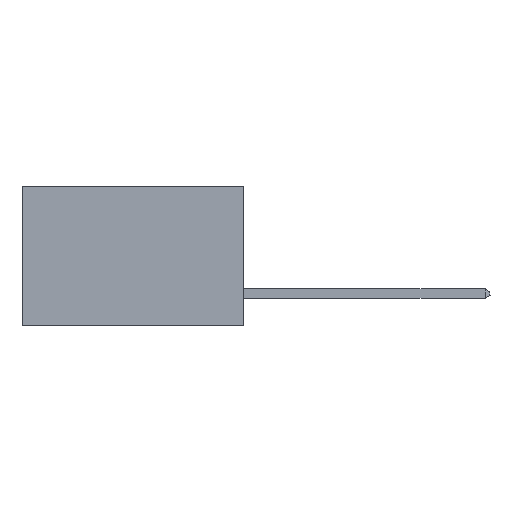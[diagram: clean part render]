
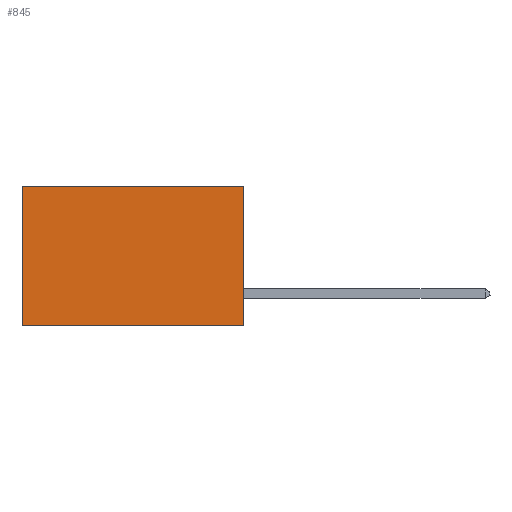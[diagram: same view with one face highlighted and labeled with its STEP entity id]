
A CAD part, left-side view. The second image highlights one B-rep face of the part: STEP entity #845.
In plain terms, the highlighted planar face has unit normal (-1, 0, 0).
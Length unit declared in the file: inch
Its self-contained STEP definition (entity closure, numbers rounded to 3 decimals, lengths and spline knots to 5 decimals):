
#101 = VECTOR ( 'NONE', #671, 39.37008 ) ;
#221 = VERTEX_POINT ( 'NONE', #7932 ) ;
#446 = FACE_OUTER_BOUND ( 'NONE', #1994, .T. ) ;
#671 = DIRECTION ( 'NONE',  ( 0., 1., 0. ) ) ;
#716 = LINE ( 'NONE', #1663, #6375 ) ;
#845 = ADVANCED_FACE ( 'NONE', ( #446 ), #2060, .F. ) ;
#1315 = CARTESIAN_POINT ( 'NONE',  ( 0.277, 0.59, 0. ) ) ;
#1663 = CARTESIAN_POINT ( 'NONE',  ( 0.277, 0., -0.37 ) ) ;
#1927 = VERTEX_POINT ( 'NONE', #1315 ) ;
#1994 = EDGE_LOOP ( 'NONE', ( #8398, #6626, #5329, #5713 ) ) ;
#2060 = PLANE ( 'NONE',  #7306 ) ;
#2356 = VECTOR ( 'NONE', #9151, 39.37008 ) ;
#2360 = CARTESIAN_POINT ( 'NONE',  ( 0.277, 0., -0.37 ) ) ;
#2912 = EDGE_CURVE ( 'NONE', #1927, #4018, #4092, .T. ) ;
#2963 = CARTESIAN_POINT ( 'NONE',  ( 0.277, 0., 0. ) ) ;
#3100 = VECTOR ( 'NONE', #7412, 39.37008 ) ;
#4018 = VERTEX_POINT ( 'NONE', #8126 ) ;
#4092 = LINE ( 'NONE', #9159, #2356 ) ;
#4157 = LINE ( 'NONE', #2963, #101 ) ;
#4653 = CARTESIAN_POINT ( 'NONE',  ( 0.277, 0., -0.37 ) ) ;
#5031 = LINE ( 'NONE', #2360, #3100 ) ;
#5266 = DIRECTION ( 'NONE',  ( 0., 1., 0. ) ) ;
#5329 = ORIENTED_EDGE ( 'NONE', *, *, #9054, .F. ) ;
#5713 = ORIENTED_EDGE ( 'NONE', *, *, #8326, .T. ) ;
#6375 = VECTOR ( 'NONE', #5266, 39.37008 ) ;
#6626 = ORIENTED_EDGE ( 'NONE', *, *, #8484, .F. ) ;
#7306 = AXIS2_PLACEMENT_3D ( 'NONE', #7375, #8770, #9019 ) ;
#7375 = CARTESIAN_POINT ( 'NONE',  ( 0.277, 0., -0.37 ) ) ;
#7412 = DIRECTION ( 'NONE',  ( 0., 0., -1. ) ) ;
#7932 = CARTESIAN_POINT ( 'NONE',  ( 0.277, 0., 0. ) ) ;
#8126 = CARTESIAN_POINT ( 'NONE',  ( 0.277, 0.59, -0.37 ) ) ;
#8326 = EDGE_CURVE ( 'NONE', #221, #1927, #4157, .T. ) ;
#8398 = ORIENTED_EDGE ( 'NONE', *, *, #2912, .T. ) ;
#8484 = EDGE_CURVE ( 'NONE', #9120, #4018, #716, .T. ) ;
#8770 = DIRECTION ( 'NONE',  ( 1., 0., 0. ) ) ;
#9019 = DIRECTION ( 'NONE',  ( 0., 0., -1. ) ) ;
#9054 = EDGE_CURVE ( 'NONE', #221, #9120, #5031, .T. ) ;
#9120 = VERTEX_POINT ( 'NONE', #4653 ) ;
#9151 = DIRECTION ( 'NONE',  ( 0., 0., -1. ) ) ;
#9159 = CARTESIAN_POINT ( 'NONE',  ( 0.277, 0.59, -0.37 ) ) ;
